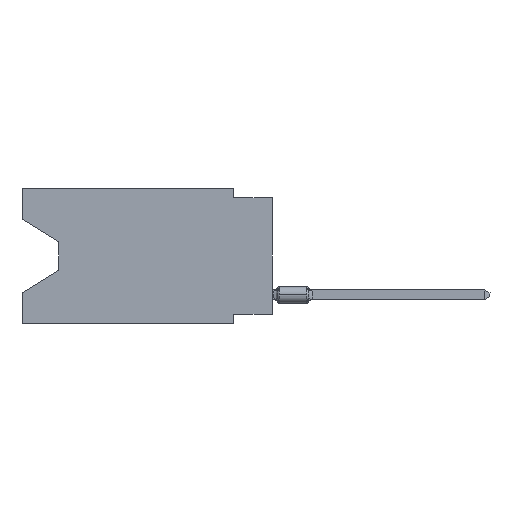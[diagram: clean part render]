
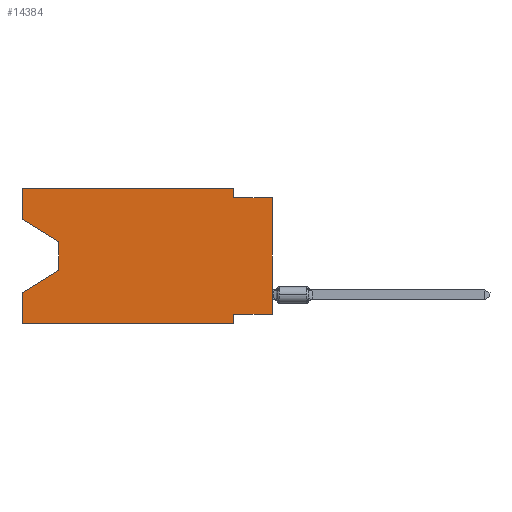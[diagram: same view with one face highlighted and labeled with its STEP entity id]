
A CAD part, left-side view. The second image highlights one B-rep face of the part: STEP entity #14384.
In plain terms, the highlighted planar face has unit normal (-1, 0, 0).
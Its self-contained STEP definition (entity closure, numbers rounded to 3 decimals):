
#183 = CARTESIAN_POINT ( 'NONE',  ( 0., 16.383, -8.89 ) ) ;
#270 = VERTEX_POINT ( 'NONE', #18726 ) ;
#494 = LINE ( 'NONE', #908, #6042 ) ;
#559 = ORIENTED_EDGE ( 'NONE', *, *, #14290, .F. ) ;
#908 = CARTESIAN_POINT ( 'NONE',  ( 0., 16.383, 0. ) ) ;
#1837 = ORIENTED_EDGE ( 'NONE', *, *, #19305, .F. ) ;
#2112 = DIRECTION ( 'NONE',  ( 1., 0., 0. ) ) ;
#2417 = EDGE_CURVE ( 'NONE', #7252, #24954, #12823, .T. ) ;
#3368 = CARTESIAN_POINT ( 'NONE',  ( 0., 0., 0. ) ) ;
#4074 = DIRECTION ( 'NONE',  ( 0., 0., 1. ) ) ;
#4208 = VERTEX_POINT ( 'NONE', #183 ) ;
#4418 = DIRECTION ( 'NONE',  ( 0., 0., -1. ) ) ;
#4971 = CARTESIAN_POINT ( 'NONE',  ( 0., 13.97, -3.505 ) ) ;
#5021 = EDGE_LOOP ( 'NONE', ( #10051, #6036, #8764, #7323, #19727, #559, #9321, #22902, #13374, #23675, #1837, #20986 ) ) ;
#5071 = CARTESIAN_POINT ( 'NONE',  ( 0., 16.383, -8.89 ) ) ;
#5077 = DIRECTION ( 'NONE',  ( 0., 0., 1. ) ) ;
#5360 = LINE ( 'NONE', #5071, #26137 ) ;
#5541 = CARTESIAN_POINT ( 'NONE',  ( 0., 2.54, 0. ) ) ;
#6036 = ORIENTED_EDGE ( 'NONE', *, *, #8963, .T. ) ;
#6042 = VECTOR ( 'NONE', #6495, 1000. ) ;
#6249 = DIRECTION ( 'NONE',  ( 0., -0.855, -0.519 ) ) ;
#6495 = DIRECTION ( 'NONE',  ( 0., -1., 0. ) ) ;
#6513 = LINE ( 'NONE', #21761, #23347 ) ;
#6518 = CARTESIAN_POINT ( 'NONE',  ( 0., 16.383, -2.038 ) ) ;
#6600 = VECTOR ( 'NONE', #17478, 1000. ) ;
#7001 = EDGE_CURVE ( 'NONE', #7252, #26342, #14724, .T. ) ;
#7252 = VERTEX_POINT ( 'NONE', #9667 ) ;
#7261 = EDGE_CURVE ( 'NONE', #15245, #8193, #16208, .T. ) ;
#7323 = ORIENTED_EDGE ( 'NONE', *, *, #19562, .F. ) ;
#7459 = VECTOR ( 'NONE', #18513, 1000. ) ;
#7984 = VECTOR ( 'NONE', #4418, 1000. ) ;
#8193 = VERTEX_POINT ( 'NONE', #25372 ) ;
#8456 = VERTEX_POINT ( 'NONE', #15575 ) ;
#8764 = ORIENTED_EDGE ( 'NONE', *, *, #9362, .T. ) ;
#8963 = EDGE_CURVE ( 'NONE', #26342, #16320, #23668, .T. ) ;
#9010 = CARTESIAN_POINT ( 'NONE',  ( 0., 13.97, -5.385 ) ) ;
#9321 = ORIENTED_EDGE ( 'NONE', *, *, #14832, .F. ) ;
#9362 = EDGE_CURVE ( 'NONE', #16320, #270, #23600, .T. ) ;
#9667 = CARTESIAN_POINT ( 'NONE',  ( 0., 16.383, -2.038 ) ) ;
#9927 = DIRECTION ( 'NONE',  ( 0., 0., 1. ) ) ;
#10051 = ORIENTED_EDGE ( 'NONE', *, *, #7001, .T. ) ;
#10450 = DIRECTION ( 'NONE',  ( 0., 0., -1. ) ) ;
#11457 = VECTOR ( 'NONE', #6249, 1000. ) ;
#11607 = CARTESIAN_POINT ( 'NONE',  ( 0., 16.383, 0. ) ) ;
#12047 = CARTESIAN_POINT ( 'NONE',  ( 0., 13.97, -3.505 ) ) ;
#12217 = CARTESIAN_POINT ( 'NONE',  ( 0., 0., -8.255 ) ) ;
#12502 = FACE_OUTER_BOUND ( 'NONE', #5021, .T. ) ;
#12823 = LINE ( 'NONE', #25207, #21689 ) ;
#13374 = ORIENTED_EDGE ( 'NONE', *, *, #18025, .F. ) ;
#13702 = DIRECTION ( 'NONE',  ( 0., -1., 0. ) ) ;
#13732 = DIRECTION ( 'NONE',  ( 0., 0., -1. ) ) ;
#14173 = CARTESIAN_POINT ( 'NONE',  ( 0., 0., -0.635 ) ) ;
#14186 = CARTESIAN_POINT ( 'NONE',  ( 0., 2.54, -8.255 ) ) ;
#14259 = LINE ( 'NONE', #12217, #18313 ) ;
#14290 = EDGE_CURVE ( 'NONE', #21464, #8456, #18497, .T. ) ;
#14384 = ADVANCED_FACE ( 'NONE', ( #12502 ), #20802, .F. ) ;
#14724 = LINE ( 'NONE', #6518, #11457 ) ;
#14832 = EDGE_CURVE ( 'NONE', #15245, #21464, #14259, .T. ) ;
#15004 = EDGE_CURVE ( 'NONE', #4208, #8456, #5360, .T. ) ;
#15245 = VERTEX_POINT ( 'NONE', #26489 ) ;
#15469 = CARTESIAN_POINT ( 'NONE',  ( 0., 16.383, 0. ) ) ;
#15575 = CARTESIAN_POINT ( 'NONE',  ( 0., 2.54, -8.89 ) ) ;
#16208 = LINE ( 'NONE', #3368, #17580 ) ;
#16213 = LINE ( 'NONE', #14173, #7459 ) ;
#16320 = VERTEX_POINT ( 'NONE', #20710 ) ;
#16455 = CARTESIAN_POINT ( 'NONE',  ( 0., 16.383, 0. ) ) ;
#16973 = VECTOR ( 'NONE', #5077, 1000. ) ;
#17478 = DIRECTION ( 'NONE',  ( 0., 0.855, -0.519 ) ) ;
#17580 = VECTOR ( 'NONE', #9927, 1000. ) ;
#18025 = EDGE_CURVE ( 'NONE', #19340, #8193, #16213, .T. ) ;
#18313 = VECTOR ( 'NONE', #20119, 1000. ) ;
#18497 = LINE ( 'NONE', #22841, #20462 ) ;
#18513 = DIRECTION ( 'NONE',  ( 0., -1., 0. ) ) ;
#18726 = CARTESIAN_POINT ( 'NONE',  ( 0., 16.383, -6.852 ) ) ;
#19277 = LINE ( 'NONE', #15469, #16973 ) ;
#19305 = EDGE_CURVE ( 'NONE', #24954, #24330, #494, .T. ) ;
#19340 = VERTEX_POINT ( 'NONE', #21503 ) ;
#19562 = EDGE_CURVE ( 'NONE', #4208, #270, #19277, .T. ) ;
#19727 = ORIENTED_EDGE ( 'NONE', *, *, #15004, .T. ) ;
#20119 = DIRECTION ( 'NONE',  ( 0., 1., 0. ) ) ;
#20462 = VECTOR ( 'NONE', #26686, 1000. ) ;
#20710 = CARTESIAN_POINT ( 'NONE',  ( 0., 13.97, -5.385 ) ) ;
#20802 = PLANE ( 'NONE',  #23932 ) ;
#20986 = ORIENTED_EDGE ( 'NONE', *, *, #2417, .F. ) ;
#21464 = VERTEX_POINT ( 'NONE', #14186 ) ;
#21503 = CARTESIAN_POINT ( 'NONE',  ( 0., 2.54, -0.635 ) ) ;
#21689 = VECTOR ( 'NONE', #4074, 1000. ) ;
#21761 = CARTESIAN_POINT ( 'NONE',  ( 0., 2.54, 0. ) ) ;
#22841 = CARTESIAN_POINT ( 'NONE',  ( 0., 2.54, -8.89 ) ) ;
#22902 = ORIENTED_EDGE ( 'NONE', *, *, #7261, .T. ) ;
#23321 = EDGE_CURVE ( 'NONE', #24330, #19340, #6513, .T. ) ;
#23347 = VECTOR ( 'NONE', #13732, 1000. ) ;
#23600 = LINE ( 'NONE', #9010, #6600 ) ;
#23668 = LINE ( 'NONE', #4971, #7984 ) ;
#23675 = ORIENTED_EDGE ( 'NONE', *, *, #23321, .F. ) ;
#23932 = AXIS2_PLACEMENT_3D ( 'NONE', #16455, #2112, #10450 ) ;
#24330 = VERTEX_POINT ( 'NONE', #5541 ) ;
#24954 = VERTEX_POINT ( 'NONE', #11607 ) ;
#25207 = CARTESIAN_POINT ( 'NONE',  ( 0., 16.383, 0. ) ) ;
#25372 = CARTESIAN_POINT ( 'NONE',  ( 0., 0., -0.635 ) ) ;
#26137 = VECTOR ( 'NONE', #13702, 1000. ) ;
#26342 = VERTEX_POINT ( 'NONE', #12047 ) ;
#26489 = CARTESIAN_POINT ( 'NONE',  ( 0., 0., -8.255 ) ) ;
#26686 = DIRECTION ( 'NONE',  ( 0., 0., -1. ) ) ;
